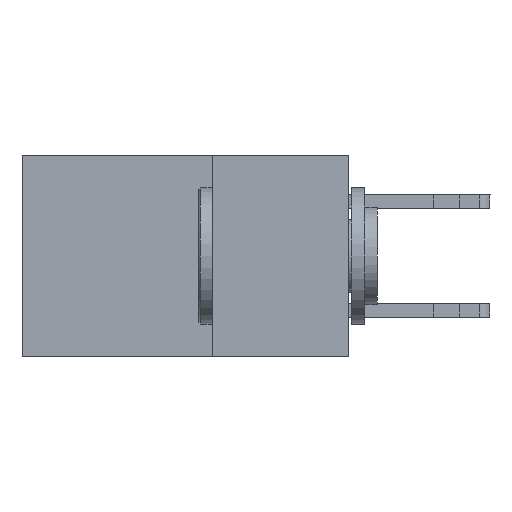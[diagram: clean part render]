
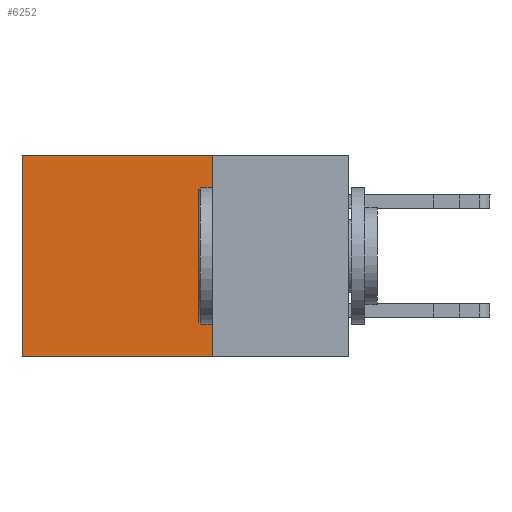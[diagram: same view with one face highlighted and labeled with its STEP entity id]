
A CAD part, left-side view. The second image highlights one B-rep face of the part: STEP entity #6252.
In plain terms, the highlighted planar face has unit normal (-1, 0, 0).
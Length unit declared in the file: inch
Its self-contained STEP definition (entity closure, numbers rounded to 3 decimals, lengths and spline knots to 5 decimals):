
#539 = EDGE_CURVE ( 'NONE', #13040, #7107, #9142, .T. ) ;
#632 = AXIS2_PLACEMENT_3D ( 'NONE', #10258, #8389, #23659 ) ;
#1237 = LINE ( 'NONE', #7396, #16758 ) ;
#1314 = DIRECTION ( 'NONE',  ( 0., 1., 0. ) ) ;
#3084 = VECTOR ( 'NONE', #1314, 39.37008 ) ;
#3305 = ORIENTED_EDGE ( 'NONE', *, *, #20457, .T. ) ;
#4354 = VERTEX_POINT ( 'NONE', #24040 ) ;
#4865 = CARTESIAN_POINT ( 'NONE',  ( 0.298, 0.6, 0. ) ) ;
#5754 = ORIENTED_EDGE ( 'NONE', *, *, #539, .F. ) ;
#6252 = ADVANCED_FACE ( 'NONE', ( #10388 ), #14041, .F. ) ;
#6321 = EDGE_CURVE ( 'NONE', #4354, #7107, #12906, .T. ) ;
#7107 = VERTEX_POINT ( 'NONE', #21966 ) ;
#7396 = CARTESIAN_POINT ( 'NONE',  ( 0.298, 0.25, 0. ) ) ;
#7489 = EDGE_LOOP ( 'NONE', ( #12256, #5754, #23621, #3305 ) ) ;
#8389 = DIRECTION ( 'NONE',  ( 1., 0., 0. ) ) ;
#9142 = LINE ( 'NONE', #19033, #13018 ) ;
#9695 = CARTESIAN_POINT ( 'NONE',  ( 0.298, 0.25, 0. ) ) ;
#10258 = CARTESIAN_POINT ( 'NONE',  ( 0.298, 0.25, 0. ) ) ;
#10388 = FACE_OUTER_BOUND ( 'NONE', #7489, .T. ) ;
#10464 = CARTESIAN_POINT ( 'NONE',  ( 0.298, 0.25, -0.37 ) ) ;
#12256 = ORIENTED_EDGE ( 'NONE', *, *, #6321, .T. ) ;
#12906 = LINE ( 'NONE', #4865, #15506 ) ;
#13009 = CARTESIAN_POINT ( 'NONE',  ( 0.298, 0.25, 0. ) ) ;
#13018 = VECTOR ( 'NONE', #24544, 39.37008 ) ;
#13040 = VERTEX_POINT ( 'NONE', #10464 ) ;
#14041 = PLANE ( 'NONE',  #632 ) ;
#15506 = VECTOR ( 'NONE', #18527, 39.37008 ) ;
#16758 = VECTOR ( 'NONE', #22173, 39.37008 ) ;
#18508 = LINE ( 'NONE', #13009, #3084 ) ;
#18527 = DIRECTION ( 'NONE',  ( 0., 0., -1. ) ) ;
#19033 = CARTESIAN_POINT ( 'NONE',  ( 0.298, 0.25, -0.37 ) ) ;
#20457 = EDGE_CURVE ( 'NONE', #23687, #4354, #18508, .T. ) ;
#21966 = CARTESIAN_POINT ( 'NONE',  ( 0.298, 0.6, -0.37 ) ) ;
#22173 = DIRECTION ( 'NONE',  ( 0., 0., -1. ) ) ;
#22203 = EDGE_CURVE ( 'NONE', #23687, #13040, #1237, .T. ) ;
#23621 = ORIENTED_EDGE ( 'NONE', *, *, #22203, .F. ) ;
#23659 = DIRECTION ( 'NONE',  ( 0., 0., -1. ) ) ;
#23687 = VERTEX_POINT ( 'NONE', #9695 ) ;
#24040 = CARTESIAN_POINT ( 'NONE',  ( 0.298, 0.6, 0. ) ) ;
#24544 = DIRECTION ( 'NONE',  ( 0., 1., 0. ) ) ;
